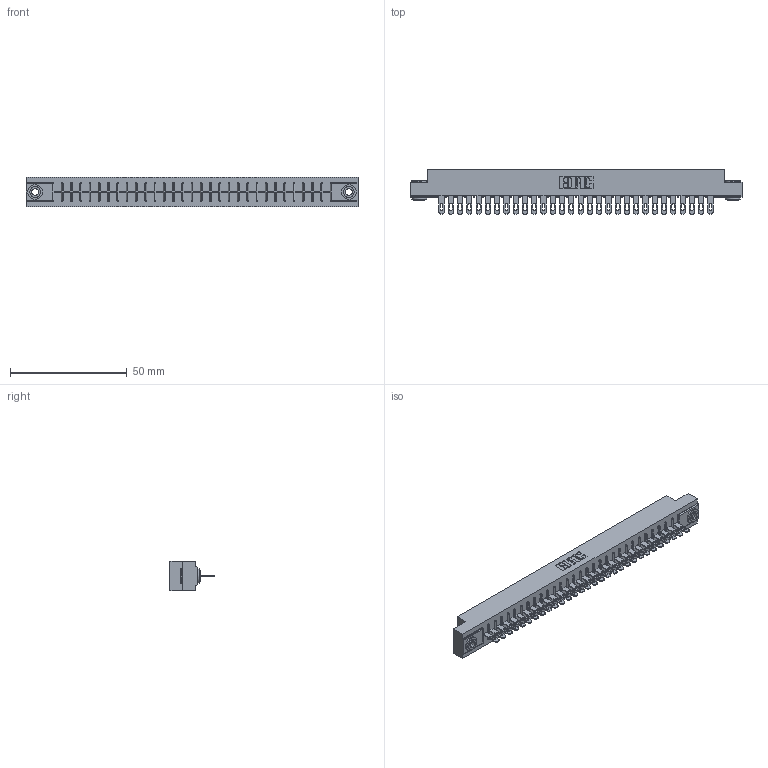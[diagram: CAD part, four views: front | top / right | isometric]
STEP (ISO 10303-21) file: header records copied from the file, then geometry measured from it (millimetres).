
FILE_DESCRIPTION (( 'STEP AP203' ), '1' );
FILE_NAME ('356-030-400-103.STEP', '2020-09-23T20:19:32', ( '' ), ( '' ), 'SwSTEP 2.0', 'SolidWorks 2020', '' );
FILE_SCHEMA (( 'CONFIG_CONTROL_DESIGN' ));
Length unit declared in the file: inch
Products named in the file (4): 306 Part_.156 Dia; 345-250-002_345-250-002-102; 306-290-001_100; 356-030-400-103
Assembly tree (33 placements, depth 2):
  356-030-400-103
    306 Part_.156 Dia
    306-290-001_100  x30
    345-250-002_345-250-002-102  x2
Bounding box: 141.88 x 18.87 x 12.7 mm (x, y, z)
Volume: 15676.2 mm3; surface area: 16747.9 mm2
Topology: 33 solids, 33 shells, 2448 faces, 6878 edges, 4420 vertices
Faces by surface type: plane 1592, cylinder 728, sphere 120, cone 8
Entity records: 30760 total; most frequent: CARTESIAN_POINT 5142, ORIENTED_EDGE 5088, DIRECTION 5086, EDGE_CURVE 2544, VECTOR 1974, LINE 1974, VERTEX_POINT 1612, AXIS2_PLACEMENT_3D 1556
